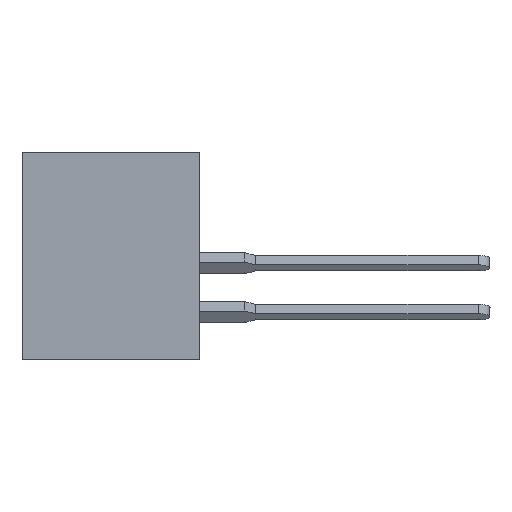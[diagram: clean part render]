
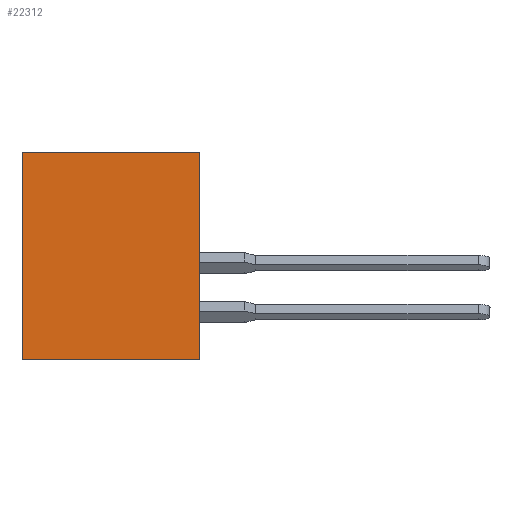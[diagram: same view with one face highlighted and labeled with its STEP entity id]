
A CAD part, left-side view. The second image highlights one B-rep face of the part: STEP entity #22312.
In plain terms, the highlighted planar face has unit normal (-1, 0, 0).
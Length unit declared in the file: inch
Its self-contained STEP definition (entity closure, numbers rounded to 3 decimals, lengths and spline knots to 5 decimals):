
#662 = CARTESIAN_POINT ( 'NONE',  ( 0., 0., 0. ) ) ;
#2877 = FACE_OUTER_BOUND ( 'NONE', #9233, .T. ) ;
#4012 = EDGE_CURVE ( 'NONE', #17442, #13862, #9745, .T. ) ;
#4313 = EDGE_CURVE ( 'NONE', #5427, #17442, #26296, .T. ) ;
#4420 = ORIENTED_EDGE ( 'NONE', *, *, #13596, .T. ) ;
#4639 = CARTESIAN_POINT ( 'NONE',  ( 0., 0.453, -0.531 ) ) ;
#5086 = VECTOR ( 'NONE', #19465, 39.37008 ) ;
#5093 = EDGE_CURVE ( 'NONE', #5427, #12253, #21999, .T. ) ;
#5427 = VERTEX_POINT ( 'NONE', #21019 ) ;
#5948 = DIRECTION ( 'NONE',  ( 0., 0., 1. ) ) ;
#7437 = DIRECTION ( 'NONE',  ( 0., 0., 1. ) ) ;
#7739 = DIRECTION ( 'NONE',  ( 0., 0., -1. ) ) ;
#7765 = VECTOR ( 'NONE', #7437, 39.37008 ) ;
#8406 = DIRECTION ( 'NONE',  ( 0., -1., 0. ) ) ;
#9044 = ORIENTED_EDGE ( 'NONE', *, *, #4012, .F. ) ;
#9233 = EDGE_LOOP ( 'NONE', ( #4420, #9044, #26645, #15958 ) ) ;
#9591 = DIRECTION ( 'NONE',  ( 1., 0., 0. ) ) ;
#9745 = LINE ( 'NONE', #16837, #24028 ) ;
#10403 = VECTOR ( 'NONE', #5948, 39.37008 ) ;
#12253 = VERTEX_POINT ( 'NONE', #21902 ) ;
#13596 = EDGE_CURVE ( 'NONE', #12253, #13862, #18363, .T. ) ;
#13862 = VERTEX_POINT ( 'NONE', #662 ) ;
#15958 = ORIENTED_EDGE ( 'NONE', *, *, #5093, .T. ) ;
#16837 = CARTESIAN_POINT ( 'NONE',  ( 0., 0.453, 0. ) ) ;
#17442 = VERTEX_POINT ( 'NONE', #24523 ) ;
#18267 = AXIS2_PLACEMENT_3D ( 'NONE', #24516, #9591, #7739 ) ;
#18363 = LINE ( 'NONE', #23010, #10403 ) ;
#18421 = PLANE ( 'NONE',  #18267 ) ;
#19465 = DIRECTION ( 'NONE',  ( 0., -1., 0. ) ) ;
#20162 = CARTESIAN_POINT ( 'NONE',  ( 0., 0.453, 0. ) ) ;
#21019 = CARTESIAN_POINT ( 'NONE',  ( 0., 0.453, -0.531 ) ) ;
#21902 = CARTESIAN_POINT ( 'NONE',  ( 0., 0., -0.531 ) ) ;
#21999 = LINE ( 'NONE', #4639, #5086 ) ;
#22312 = ADVANCED_FACE ( 'NONE', ( #2877 ), #18421, .F. ) ;
#23010 = CARTESIAN_POINT ( 'NONE',  ( 0., 0., 0. ) ) ;
#24028 = VECTOR ( 'NONE', #8406, 39.37008 ) ;
#24516 = CARTESIAN_POINT ( 'NONE',  ( 0., 0.453, 0. ) ) ;
#24523 = CARTESIAN_POINT ( 'NONE',  ( 0., 0.453, 0. ) ) ;
#26296 = LINE ( 'NONE', #20162, #7765 ) ;
#26645 = ORIENTED_EDGE ( 'NONE', *, *, #4313, .F. ) ;
